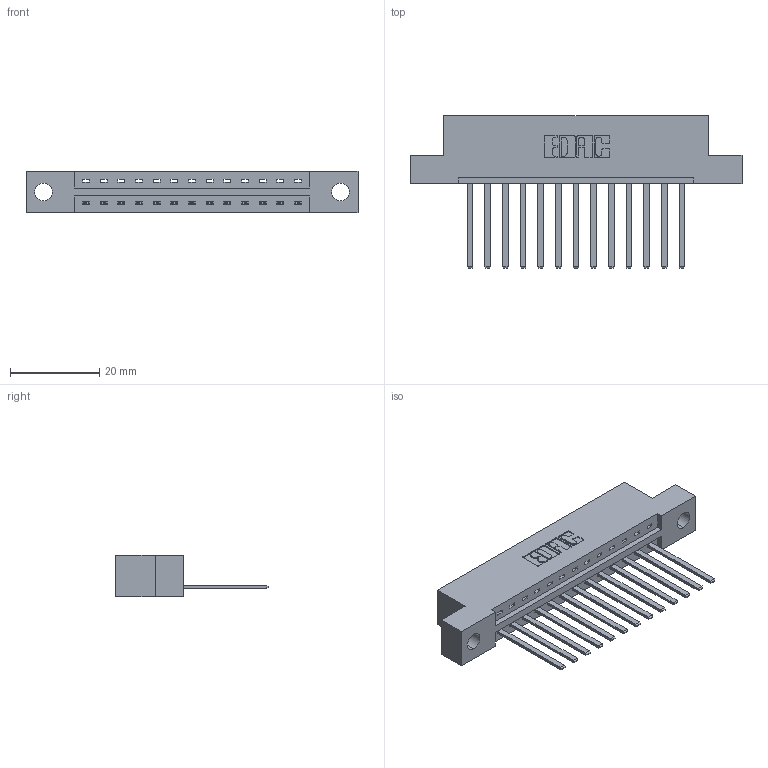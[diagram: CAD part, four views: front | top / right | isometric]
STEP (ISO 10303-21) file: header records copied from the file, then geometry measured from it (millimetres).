
FILE_DESCRIPTION (( 'STEP AP203' ), '1' );
FILE_NAME ('337-013-544-104.STEP', '2019-09-28T02:28:06', ( '' ), ( '' ), 'SwSTEP 2.0', 'SolidWorks 2016', '' );
FILE_SCHEMA (( 'CONFIG_CONTROL_DESIGN' ));
Length unit declared in the file: inch
Products named in the file (3): 345-292-001_345-293-144; 337 Part_Flush Mounting Lugs - 0.156 Dia-TH; 337-013-544-104
Assembly tree (14 placements, depth 2):
  337-013-544-104
    337 Part_Flush Mounting Lugs - 0.156 Dia-TH
    345-292-001_345-293-144  x13
Bounding box: 74.52 x 34.3 x 9.4 mm (x, y, z)
Volume: 7445.3 mm3; surface area: 7823.2 mm2
Topology: 14 solids, 14 shells, 842 faces, 2521 edges, 1662 vertices
Faces by surface type: plane 616, cylinder 226
Entity records: 13233 total; most frequent: CARTESIAN_POINT 2309, ORIENTED_EDGE 2258, DIRECTION 1999, EDGE_CURVE 1129, LINE 1005, VECTOR 1005, VERTEX_POINT 750, AXIS2_PLACEMENT_3D 497
